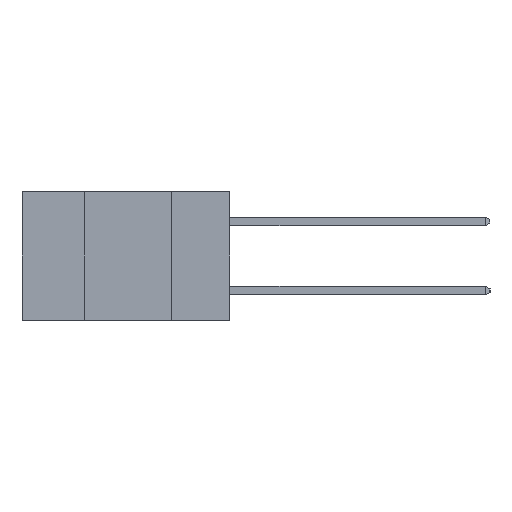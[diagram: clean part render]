
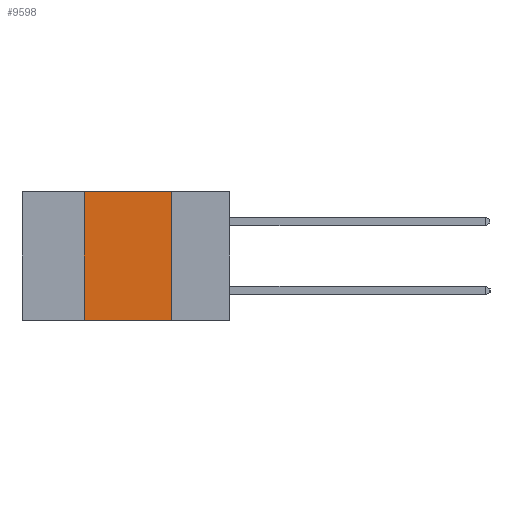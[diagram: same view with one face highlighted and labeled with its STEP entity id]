
A CAD part, left-side view. The second image highlights one B-rep face of the part: STEP entity #9598.
In plain terms, the highlighted planar face has unit normal (-1, 0, 0).
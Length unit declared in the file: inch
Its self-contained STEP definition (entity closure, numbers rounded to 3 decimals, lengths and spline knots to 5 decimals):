
#906 = DIRECTION ( 'NONE',  ( 0., 0., 1. ) ) ;
#1508 = LINE ( 'NONE', #13575, #5057 ) ;
#1585 = DIRECTION ( 'NONE',  ( 0., -1., 0. ) ) ;
#1727 = DIRECTION ( 'NONE',  ( 0., 0., -1. ) ) ;
#2553 = PLANE ( 'NONE',  #2750 ) ;
#2750 = AXIS2_PLACEMENT_3D ( 'NONE', #17361, #13016, #4064 ) ;
#2915 = LINE ( 'NONE', #18092, #8982 ) ;
#3099 = VECTOR ( 'NONE', #906, 39.37008 ) ;
#3367 = CARTESIAN_POINT ( 'NONE',  ( 0., 0.6, 0. ) ) ;
#3539 = ORIENTED_EDGE ( 'NONE', *, *, #13430, .F. ) ;
#4064 = DIRECTION ( 'NONE',  ( 0., 0., -1. ) ) ;
#5057 = VECTOR ( 'NONE', #1585, 39.37008 ) ;
#5818 = VECTOR ( 'NONE', #7784, 39.37008 ) ;
#6281 = EDGE_LOOP ( 'NONE', ( #10061, #18334, #3539, #7474 ) ) ;
#6298 = VERTEX_POINT ( 'NONE', #12569 ) ;
#7053 = LINE ( 'NONE', #18718, #3099 ) ;
#7474 = ORIENTED_EDGE ( 'NONE', *, *, #10412, .T. ) ;
#7784 = DIRECTION ( 'NONE',  ( 0., -1., 0. ) ) ;
#8982 = VECTOR ( 'NONE', #1727, 39.37008 ) ;
#9283 = EDGE_CURVE ( 'NONE', #12235, #18004, #14211, .T. ) ;
#9598 = ADVANCED_FACE ( 'NONE', ( #12105 ), #2553, .F. ) ;
#10061 = ORIENTED_EDGE ( 'NONE', *, *, #17939, .F. ) ;
#10412 = EDGE_CURVE ( 'NONE', #6298, #17865, #1508, .T. ) ;
#12105 = FACE_OUTER_BOUND ( 'NONE', #6281, .T. ) ;
#12235 = VERTEX_POINT ( 'NONE', #13360 ) ;
#12569 = CARTESIAN_POINT ( 'NONE',  ( 0., 0.42, -0.37 ) ) ;
#13016 = DIRECTION ( 'NONE',  ( 1., 0., 0. ) ) ;
#13360 = CARTESIAN_POINT ( 'NONE',  ( 0., 0.42, 0. ) ) ;
#13430 = EDGE_CURVE ( 'NONE', #6298, #12235, #7053, .T. ) ;
#13575 = CARTESIAN_POINT ( 'NONE',  ( 0., 0.6, -0.37 ) ) ;
#13819 = CARTESIAN_POINT ( 'NONE',  ( 0., 0.17, 0. ) ) ;
#14211 = LINE ( 'NONE', #3367, #5818 ) ;
#16496 = CARTESIAN_POINT ( 'NONE',  ( 0., 0.17, -0.37 ) ) ;
#17361 = CARTESIAN_POINT ( 'NONE',  ( 0., 0.6, 0. ) ) ;
#17865 = VERTEX_POINT ( 'NONE', #16496 ) ;
#17939 = EDGE_CURVE ( 'NONE', #18004, #17865, #2915, .T. ) ;
#18004 = VERTEX_POINT ( 'NONE', #13819 ) ;
#18092 = CARTESIAN_POINT ( 'NONE',  ( 0., 0.17, -0.37 ) ) ;
#18334 = ORIENTED_EDGE ( 'NONE', *, *, #9283, .F. ) ;
#18718 = CARTESIAN_POINT ( 'NONE',  ( 0., 0.42, -0.37 ) ) ;
